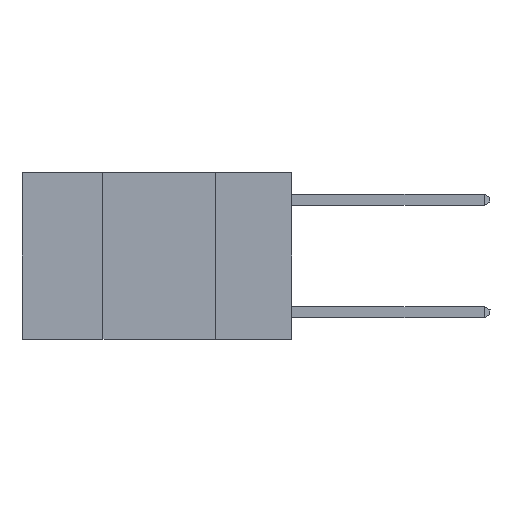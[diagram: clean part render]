
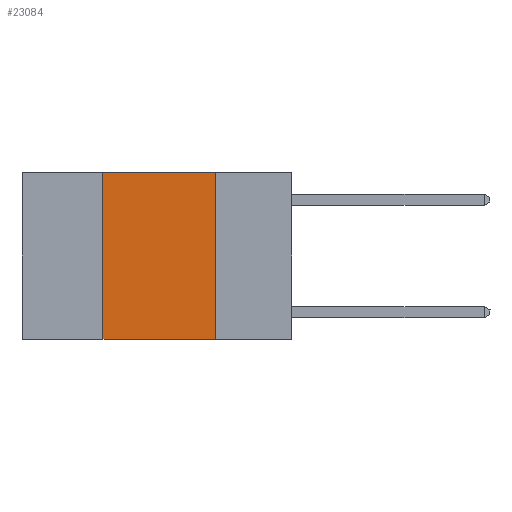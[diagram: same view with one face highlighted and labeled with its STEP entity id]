
A CAD part, left-side view. The second image highlights one B-rep face of the part: STEP entity #23084.
In plain terms, the highlighted planar face has unit normal (-1, 0, 0).
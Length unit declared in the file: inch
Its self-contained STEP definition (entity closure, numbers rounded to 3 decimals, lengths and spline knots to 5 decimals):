
#523 = CARTESIAN_POINT ( 'NONE',  ( 0., 0.6, -0.37 ) ) ;
#779 = DIRECTION ( 'NONE',  ( 0., -1., 0. ) ) ;
#942 = DIRECTION ( 'NONE',  ( 0., 0., -1. ) ) ;
#1389 = DIRECTION ( 'NONE',  ( 0., -1., 0. ) ) ;
#1569 = EDGE_CURVE ( 'NONE', #4084, #24169, #25479, .T. ) ;
#1827 = CARTESIAN_POINT ( 'NONE',  ( 0., 0.17, 0. ) ) ;
#3227 = VECTOR ( 'NONE', #779, 39.37008 ) ;
#4011 = ORIENTED_EDGE ( 'NONE', *, *, #5321, .F. ) ;
#4084 = VERTEX_POINT ( 'NONE', #7244 ) ;
#5321 = EDGE_CURVE ( 'NONE', #4084, #23278, #16304, .T. ) ;
#7244 = CARTESIAN_POINT ( 'NONE',  ( 0., 0.42, -0.37 ) ) ;
#7862 = DIRECTION ( 'NONE',  ( 0., 0., -1. ) ) ;
#8218 = VERTEX_POINT ( 'NONE', #25018 ) ;
#9502 = VECTOR ( 'NONE', #1389, 39.37008 ) ;
#9534 = CARTESIAN_POINT ( 'NONE',  ( 0., 0.42, 0. ) ) ;
#10274 = CARTESIAN_POINT ( 'NONE',  ( 0., 0.17, -0.37 ) ) ;
#11033 = CARTESIAN_POINT ( 'NONE',  ( 0., 0.6, 0. ) ) ;
#11175 = EDGE_CURVE ( 'NONE', #23278, #8218, #24000, .T. ) ;
#12903 = CARTESIAN_POINT ( 'NONE',  ( 0., 0.42, 0. ) ) ;
#12920 = CARTESIAN_POINT ( 'NONE',  ( 0., 0.6, 0. ) ) ;
#13064 = AXIS2_PLACEMENT_3D ( 'NONE', #11033, #13080, #942 ) ;
#13080 = DIRECTION ( 'NONE',  ( 1., 0., 0. ) ) ;
#14366 = LINE ( 'NONE', #1827, #24987 ) ;
#14931 = DIRECTION ( 'NONE',  ( 0., 0., 1. ) ) ;
#16304 = LINE ( 'NONE', #12903, #16939 ) ;
#16695 = FACE_OUTER_BOUND ( 'NONE', #23961, .T. ) ;
#16939 = VECTOR ( 'NONE', #14931, 39.37008 ) ;
#18670 = EDGE_CURVE ( 'NONE', #8218, #24169, #14366, .T. ) ;
#18970 = ORIENTED_EDGE ( 'NONE', *, *, #11175, .F. ) ;
#22790 = ORIENTED_EDGE ( 'NONE', *, *, #18670, .F. ) ;
#23084 = ADVANCED_FACE ( 'NONE', ( #16695 ), #25038, .F. ) ;
#23278 = VERTEX_POINT ( 'NONE', #9534 ) ;
#23360 = ORIENTED_EDGE ( 'NONE', *, *, #1569, .T. ) ;
#23961 = EDGE_LOOP ( 'NONE', ( #22790, #18970, #4011, #23360 ) ) ;
#24000 = LINE ( 'NONE', #12920, #3227 ) ;
#24169 = VERTEX_POINT ( 'NONE', #10274 ) ;
#24987 = VECTOR ( 'NONE', #7862, 39.37008 ) ;
#25018 = CARTESIAN_POINT ( 'NONE',  ( 0., 0.17, 0. ) ) ;
#25038 = PLANE ( 'NONE',  #13064 ) ;
#25479 = LINE ( 'NONE', #523, #9502 ) ;
